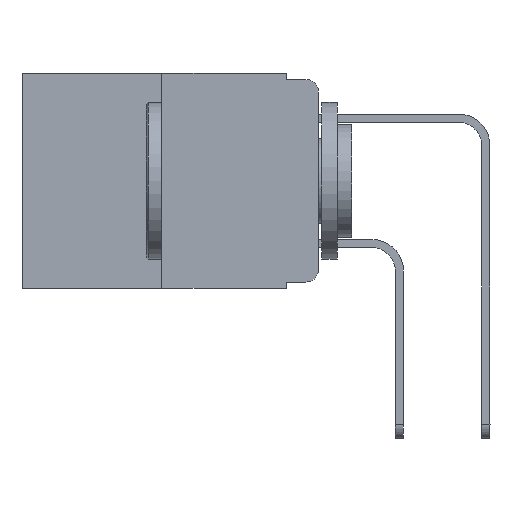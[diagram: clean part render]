
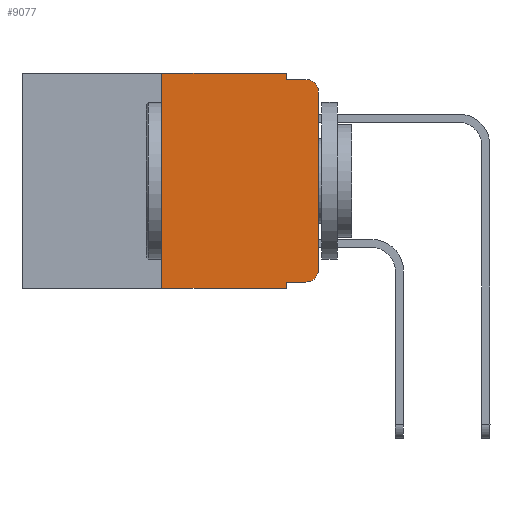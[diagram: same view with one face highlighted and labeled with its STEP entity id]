
A CAD part, left-side view. The second image highlights one B-rep face of the part: STEP entity #9077.
In plain terms, the highlighted planar face has unit normal (-1, 0, 0).
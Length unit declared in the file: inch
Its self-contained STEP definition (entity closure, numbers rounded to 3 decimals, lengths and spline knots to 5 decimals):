
#564 = DIRECTION ( 'NONE',  ( 0., 0., -1. ) ) ;
#764 = DIRECTION ( 'NONE',  ( 0., 0., -1. ) ) ;
#1129 = AXIS2_PLACEMENT_3D ( 'NONE', #5872, #16951, #11645 ) ;
#1781 = AXIS2_PLACEMENT_3D ( 'NONE', #15187, #2557, #11553 ) ;
#2248 = CARTESIAN_POINT ( 'NONE',  ( 0., 0.02, -0.313 ) ) ;
#2557 = DIRECTION ( 'NONE',  ( 1., 0., 0. ) ) ;
#2621 = CARTESIAN_POINT ( 'NONE',  ( 0., 0.25, -0.343 ) ) ;
#2705 = VECTOR ( 'NONE', #6643, 39.37008 ) ;
#2806 = VERTEX_POINT ( 'NONE', #16701 ) ;
#2893 = CARTESIAN_POINT ( 'NONE',  ( 0., 0.051, -0.333 ) ) ;
#3004 = CARTESIAN_POINT ( 'NONE',  ( 0., 0.473, -0.343 ) ) ;
#3093 = LINE ( 'NONE', #10429, #5573 ) ;
#3155 = VERTEX_POINT ( 'NONE', #7495 ) ;
#3256 = DIRECTION ( 'NONE',  ( 0., 0., 1. ) ) ;
#3787 = LINE ( 'NONE', #14756, #22736 ) ;
#3811 = VECTOR ( 'NONE', #10228, 39.37008 ) ;
#4634 = VECTOR ( 'NONE', #13811, 39.37008 ) ;
#4699 = LINE ( 'NONE', #16020, #8001 ) ;
#5212 = VERTEX_POINT ( 'NONE', #5518 ) ;
#5238 = ORIENTED_EDGE ( 'NONE', *, *, #6113, .F. ) ;
#5336 = CARTESIAN_POINT ( 'NONE',  ( 0., 0.051, 0. ) ) ;
#5466 = ORIENTED_EDGE ( 'NONE', *, *, #10397, .T. ) ;
#5518 = CARTESIAN_POINT ( 'NONE',  ( 0., 0.02, -0.01 ) ) ;
#5573 = VECTOR ( 'NONE', #8617, 39.37008 ) ;
#5872 = CARTESIAN_POINT ( 'NONE',  ( 0., 0.02, -0.03 ) ) ;
#6113 = EDGE_CURVE ( 'NONE', #8885, #6452, #21253, .T. ) ;
#6436 = CARTESIAN_POINT ( 'NONE',  ( 0., 0.051, 0. ) ) ;
#6446 = CARTESIAN_POINT ( 'NONE',  ( 0., 0., 0. ) ) ;
#6452 = VERTEX_POINT ( 'NONE', #13009 ) ;
#6643 = DIRECTION ( 'NONE',  ( 0., -1., 0. ) ) ;
#7406 = EDGE_CURVE ( 'NONE', #12074, #8885, #19206, .T. ) ;
#7495 = CARTESIAN_POINT ( 'NONE',  ( 0., 0., -0.313 ) ) ;
#7543 = CARTESIAN_POINT ( 'NONE',  ( 0., 0.25, 0. ) ) ;
#8001 = VECTOR ( 'NONE', #3256, 39.37008 ) ;
#8046 = ORIENTED_EDGE ( 'NONE', *, *, #15389, .T. ) ;
#8617 = DIRECTION ( 'NONE',  ( 0., -1., 0. ) ) ;
#8708 = VECTOR ( 'NONE', #18590, 39.37008 ) ;
#8885 = VERTEX_POINT ( 'NONE', #6436 ) ;
#9077 = ADVANCED_FACE ( 'NONE', ( #9399 ), #12693, .F. ) ;
#9156 = EDGE_CURVE ( 'NONE', #23460, #20111, #21879, .T. ) ;
#9399 = FACE_OUTER_BOUND ( 'NONE', #22407, .T. ) ;
#9818 = LINE ( 'NONE', #6446, #4634 ) ;
#10228 = DIRECTION ( 'NONE',  ( 0., -1., 0. ) ) ;
#10397 = EDGE_CURVE ( 'NONE', #18882, #20111, #21221, .T. ) ;
#10429 = CARTESIAN_POINT ( 'NONE',  ( 0., 0.051, -0.01 ) ) ;
#11553 = DIRECTION ( 'NONE',  ( 0., 0., -1. ) ) ;
#11645 = DIRECTION ( 'NONE',  ( 0., 0., -1. ) ) ;
#11767 = EDGE_CURVE ( 'NONE', #18882, #12074, #4699, .T. ) ;
#12050 = EDGE_CURVE ( 'NONE', #22587, #5212, #22287, .T. ) ;
#12074 = VERTEX_POINT ( 'NONE', #7543 ) ;
#12497 = AXIS2_PLACEMENT_3D ( 'NONE', #2248, #22706, #564 ) ;
#12693 = PLANE ( 'NONE',  #1781 ) ;
#13009 = CARTESIAN_POINT ( 'NONE',  ( 0., 0.051, -0.01 ) ) ;
#13646 = CARTESIAN_POINT ( 'NONE',  ( 0., 0.051, 0. ) ) ;
#13811 = DIRECTION ( 'NONE',  ( 0., 0., 1. ) ) ;
#13817 = EDGE_CURVE ( 'NONE', #3155, #22587, #9818, .T. ) ;
#14120 = ORIENTED_EDGE ( 'NONE', *, *, #7406, .F. ) ;
#14687 = ORIENTED_EDGE ( 'NONE', *, *, #20384, .F. ) ;
#14756 = CARTESIAN_POINT ( 'NONE',  ( 0., 0.051, -0.333 ) ) ;
#15187 = CARTESIAN_POINT ( 'NONE',  ( 0., 0.473, 0. ) ) ;
#15231 = DIRECTION ( 'NONE',  ( 0., -1., 0. ) ) ;
#15389 = EDGE_CURVE ( 'NONE', #23460, #2806, #3787, .T. ) ;
#15569 = CARTESIAN_POINT ( 'NONE',  ( 0., 0.473, 0. ) ) ;
#16020 = CARTESIAN_POINT ( 'NONE',  ( 0., 0.25, 0. ) ) ;
#16346 = ORIENTED_EDGE ( 'NONE', *, *, #13817, .T. ) ;
#16701 = CARTESIAN_POINT ( 'NONE',  ( 0., 0.02, -0.333 ) ) ;
#16951 = DIRECTION ( 'NONE',  ( -1., 0., 0. ) ) ;
#17980 = ORIENTED_EDGE ( 'NONE', *, *, #11767, .F. ) ;
#18423 = CARTESIAN_POINT ( 'NONE',  ( 0., 0.051, -0.343 ) ) ;
#18590 = DIRECTION ( 'NONE',  ( 0., 0., -1. ) ) ;
#18882 = VERTEX_POINT ( 'NONE', #2621 ) ;
#19102 = ORIENTED_EDGE ( 'NONE', *, *, #12050, .T. ) ;
#19206 = LINE ( 'NONE', #15569, #2705 ) ;
#20111 = VERTEX_POINT ( 'NONE', #18423 ) ;
#20384 = EDGE_CURVE ( 'NONE', #6452, #5212, #3093, .T. ) ;
#20611 = EDGE_CURVE ( 'NONE', #2806, #3155, #20961, .T. ) ;
#20657 = VECTOR ( 'NONE', #764, 39.37008 ) ;
#20778 = CARTESIAN_POINT ( 'NONE',  ( 0., 0., -0.03 ) ) ;
#20939 = ORIENTED_EDGE ( 'NONE', *, *, #20611, .T. ) ;
#20961 = CIRCLE ( 'NONE', #12497, 0.02 ) ;
#21221 = LINE ( 'NONE', #3004, #3811 ) ;
#21253 = LINE ( 'NONE', #13646, #20657 ) ;
#21879 = LINE ( 'NONE', #5336, #8708 ) ;
#22287 = CIRCLE ( 'NONE', #1129, 0.02 ) ;
#22407 = EDGE_LOOP ( 'NONE', ( #16346, #19102, #14687, #5238, #14120, #17980, #5466, #23609, #8046, #20939 ) ) ;
#22587 = VERTEX_POINT ( 'NONE', #20778 ) ;
#22706 = DIRECTION ( 'NONE',  ( -1., 0., 0. ) ) ;
#22736 = VECTOR ( 'NONE', #15231, 39.37008 ) ;
#23460 = VERTEX_POINT ( 'NONE', #2893 ) ;
#23609 = ORIENTED_EDGE ( 'NONE', *, *, #9156, .F. ) ;
